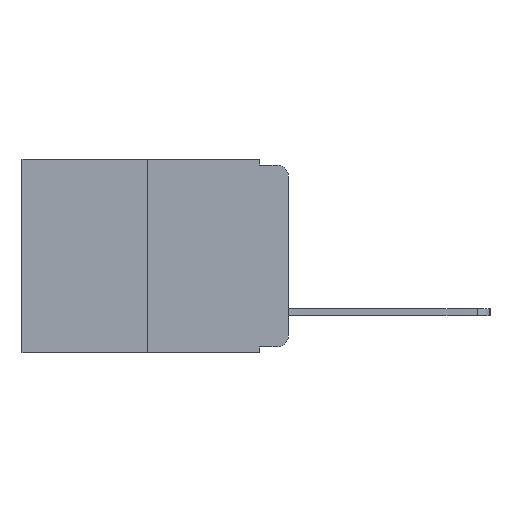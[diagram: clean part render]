
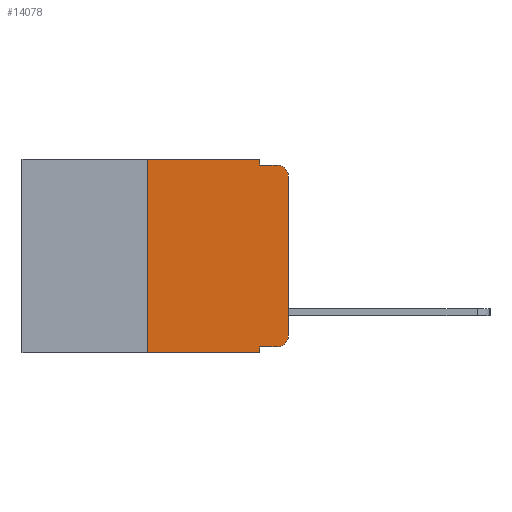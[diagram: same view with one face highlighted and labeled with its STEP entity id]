
A CAD part, left-side view. The second image highlights one B-rep face of the part: STEP entity #14078.
In plain terms, the highlighted planar face has unit normal (-1, 0, 0).
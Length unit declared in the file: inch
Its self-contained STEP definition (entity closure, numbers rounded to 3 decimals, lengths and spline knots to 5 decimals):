
#621 = VECTOR ( 'NONE', #4825, 39.37008 ) ;
#899 = ORIENTED_EDGE ( 'NONE', *, *, #14663, .T. ) ;
#1650 = EDGE_LOOP ( 'NONE', ( #5595, #13376, #10468, #14247, #11378, #15997, #899, #5365, #9306, #17314 ) ) ;
#2342 = CARTESIAN_POINT ( 'NONE',  ( 0., 0., -0.313 ) ) ;
#2812 = CARTESIAN_POINT ( 'NONE',  ( 0., 0.051, -0.01 ) ) ;
#3382 = VECTOR ( 'NONE', #14906, 39.37008 ) ;
#3434 = LINE ( 'NONE', #15515, #14678 ) ;
#3850 = LINE ( 'NONE', #6238, #3382 ) ;
#4608 = LINE ( 'NONE', #7764, #621 ) ;
#4825 = DIRECTION ( 'NONE',  ( 0., -1., 0. ) ) ;
#5004 = CARTESIAN_POINT ( 'NONE',  ( 0., 0.473, 0. ) ) ;
#5245 = CARTESIAN_POINT ( 'NONE',  ( 0., 0., -0.03 ) ) ;
#5300 = CARTESIAN_POINT ( 'NONE',  ( 0., 0.051, -0.01 ) ) ;
#5328 = CARTESIAN_POINT ( 'NONE',  ( 0., 0.25, 0. ) ) ;
#5365 = ORIENTED_EDGE ( 'NONE', *, *, #13181, .F. ) ;
#5595 = ORIENTED_EDGE ( 'NONE', *, *, #10115, .T. ) ;
#5820 = CARTESIAN_POINT ( 'NONE',  ( 0., 0.02, -0.313 ) ) ;
#5880 = LINE ( 'NONE', #15682, #13185 ) ;
#6238 = CARTESIAN_POINT ( 'NONE',  ( 0., 0., 0. ) ) ;
#6250 = LINE ( 'NONE', #15094, #10639 ) ;
#6432 = DIRECTION ( 'NONE',  ( 0., 0., 1. ) ) ;
#6440 = CIRCLE ( 'NONE', #13645, 0.02 ) ;
#6582 = VERTEX_POINT ( 'NONE', #6869 ) ;
#6764 = EDGE_CURVE ( 'NONE', #16922, #12506, #6440, .T. ) ;
#6859 = CARTESIAN_POINT ( 'NONE',  ( 0., 0.02, -0.03 ) ) ;
#6869 = CARTESIAN_POINT ( 'NONE',  ( 0., 0.051, -0.333 ) ) ;
#7124 = VERTEX_POINT ( 'NONE', #9611 ) ;
#7304 = CIRCLE ( 'NONE', #7834, 0.02 ) ;
#7316 = DIRECTION ( 'NONE',  ( 0., 0., -1. ) ) ;
#7764 = CARTESIAN_POINT ( 'NONE',  ( 0., 0.473, -0.343 ) ) ;
#7834 = AXIS2_PLACEMENT_3D ( 'NONE', #6859, #16873, #8323 ) ;
#7907 = FACE_OUTER_BOUND ( 'NONE', #1650, .T. ) ;
#7992 = PLANE ( 'NONE',  #8512 ) ;
#8323 = DIRECTION ( 'NONE',  ( 0., 0., -1. ) ) ;
#8512 = AXIS2_PLACEMENT_3D ( 'NONE', #5004, #17967, #9479 ) ;
#8514 = CARTESIAN_POINT ( 'NONE',  ( 0., 0.051, 0. ) ) ;
#8955 = LINE ( 'NONE', #8514, #13275 ) ;
#9116 = EDGE_CURVE ( 'NONE', #18420, #16724, #7304, .T. ) ;
#9147 = CARTESIAN_POINT ( 'NONE',  ( 0., 0.051, -0.333 ) ) ;
#9306 = ORIENTED_EDGE ( 'NONE', *, *, #13952, .T. ) ;
#9479 = DIRECTION ( 'NONE',  ( 0., 0., -1. ) ) ;
#9611 = CARTESIAN_POINT ( 'NONE',  ( 0., 0.25, -0.343 ) ) ;
#10115 = EDGE_CURVE ( 'NONE', #12506, #18420, #3850, .T. ) ;
#10231 = LINE ( 'NONE', #9147, #17303 ) ;
#10468 = ORIENTED_EDGE ( 'NONE', *, *, #12080, .F. ) ;
#10546 = VECTOR ( 'NONE', #15958, 39.37008 ) ;
#10639 = VECTOR ( 'NONE', #6432, 39.37008 ) ;
#11111 = EDGE_CURVE ( 'NONE', #13744, #13057, #8955, .T. ) ;
#11378 = ORIENTED_EDGE ( 'NONE', *, *, #18467, .F. ) ;
#11540 = CARTESIAN_POINT ( 'NONE',  ( 0., 0.051, 0. ) ) ;
#12080 = EDGE_CURVE ( 'NONE', #13057, #16724, #18463, .T. ) ;
#12506 = VERTEX_POINT ( 'NONE', #2342 ) ;
#12865 = DIRECTION ( 'NONE',  ( 0., 0., -1. ) ) ;
#13057 = VERTEX_POINT ( 'NONE', #5300 ) ;
#13181 = EDGE_CURVE ( 'NONE', #6582, #14837, #5880, .T. ) ;
#13185 = VECTOR ( 'NONE', #12865, 39.37008 ) ;
#13275 = VECTOR ( 'NONE', #18448, 39.37008 ) ;
#13376 = ORIENTED_EDGE ( 'NONE', *, *, #9116, .T. ) ;
#13582 = CARTESIAN_POINT ( 'NONE',  ( 0., 0.02, -0.333 ) ) ;
#13645 = AXIS2_PLACEMENT_3D ( 'NONE', #5820, #15912, #7316 ) ;
#13744 = VERTEX_POINT ( 'NONE', #11540 ) ;
#13952 = EDGE_CURVE ( 'NONE', #6582, #16922, #10231, .T. ) ;
#14078 = ADVANCED_FACE ( 'NONE', ( #7907 ), #7992, .F. ) ;
#14211 = VERTEX_POINT ( 'NONE', #5328 ) ;
#14247 = ORIENTED_EDGE ( 'NONE', *, *, #11111, .F. ) ;
#14510 = CARTESIAN_POINT ( 'NONE',  ( 0., 0.02, -0.01 ) ) ;
#14663 = EDGE_CURVE ( 'NONE', #7124, #14837, #4608, .T. ) ;
#14678 = VECTOR ( 'NONE', #16902, 39.37008 ) ;
#14837 = VERTEX_POINT ( 'NONE', #18104 ) ;
#14906 = DIRECTION ( 'NONE',  ( 0., 0., 1. ) ) ;
#15094 = CARTESIAN_POINT ( 'NONE',  ( 0., 0.25, 0. ) ) ;
#15515 = CARTESIAN_POINT ( 'NONE',  ( 0., 0.473, 0. ) ) ;
#15682 = CARTESIAN_POINT ( 'NONE',  ( 0., 0.051, 0. ) ) ;
#15830 = EDGE_CURVE ( 'NONE', #7124, #14211, #6250, .T. ) ;
#15912 = DIRECTION ( 'NONE',  ( -1., 0., 0. ) ) ;
#15958 = DIRECTION ( 'NONE',  ( 0., -1., 0. ) ) ;
#15997 = ORIENTED_EDGE ( 'NONE', *, *, #15830, .F. ) ;
#16261 = DIRECTION ( 'NONE',  ( 0., -1., 0. ) ) ;
#16724 = VERTEX_POINT ( 'NONE', #14510 ) ;
#16873 = DIRECTION ( 'NONE',  ( -1., 0., 0. ) ) ;
#16902 = DIRECTION ( 'NONE',  ( 0., -1., 0. ) ) ;
#16922 = VERTEX_POINT ( 'NONE', #13582 ) ;
#17303 = VECTOR ( 'NONE', #16261, 39.37008 ) ;
#17314 = ORIENTED_EDGE ( 'NONE', *, *, #6764, .T. ) ;
#17967 = DIRECTION ( 'NONE',  ( 1., 0., 0. ) ) ;
#18104 = CARTESIAN_POINT ( 'NONE',  ( 0., 0.051, -0.343 ) ) ;
#18420 = VERTEX_POINT ( 'NONE', #5245 ) ;
#18448 = DIRECTION ( 'NONE',  ( 0., 0., -1. ) ) ;
#18463 = LINE ( 'NONE', #2812, #10546 ) ;
#18467 = EDGE_CURVE ( 'NONE', #14211, #13744, #3434, .T. ) ;
